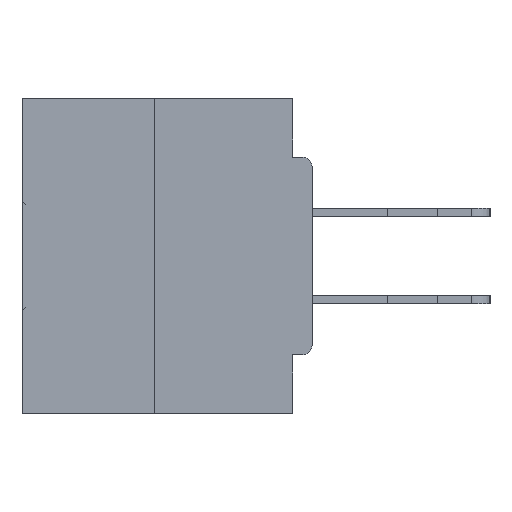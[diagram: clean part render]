
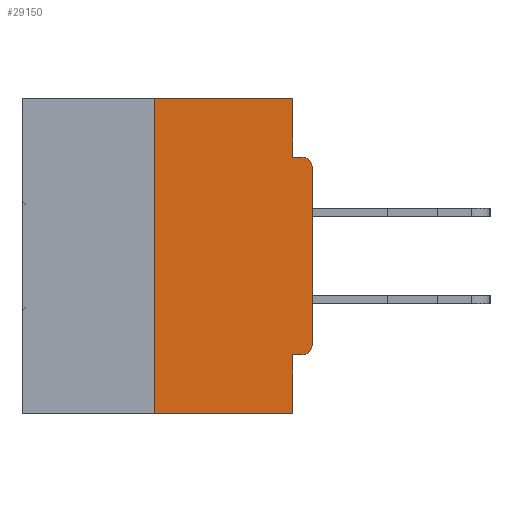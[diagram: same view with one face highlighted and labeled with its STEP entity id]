
A CAD part, left-side view. The second image highlights one B-rep face of the part: STEP entity #29150.
In plain terms, the highlighted planar face has unit normal (-1, 0, 0).
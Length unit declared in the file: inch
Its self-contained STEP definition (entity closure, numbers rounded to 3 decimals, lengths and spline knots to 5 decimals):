
#757 = DIRECTION ( 'NONE',  ( 0., -1., 0. ) ) ;
#1278 = CIRCLE ( 'NONE', #42327, 0.015 ) ;
#1602 = ORIENTED_EDGE ( 'NONE', *, *, #27210, .F. ) ;
#1636 = EDGE_CURVE ( 'NONE', #23093, #5491, #30600, .T. ) ;
#1952 = EDGE_CURVE ( 'NONE', #10516, #39162, #7034, .T. ) ;
#2072 = ORIENTED_EDGE ( 'NONE', *, *, #35229, .F. ) ;
#2387 = AXIS2_PLACEMENT_3D ( 'NONE', #27157, #37615, #17773 ) ;
#2455 = ORIENTED_EDGE ( 'NONE', *, *, #2737, .T. ) ;
#2729 = VECTOR ( 'NONE', #42596, 39.37008 ) ;
#2737 = EDGE_CURVE ( 'NONE', #21508, #10516, #1278, .T. ) ;
#2863 = VERTEX_POINT ( 'NONE', #5063 ) ;
#3002 = ORIENTED_EDGE ( 'NONE', *, *, #21280, .T. ) ;
#3651 = VERTEX_POINT ( 'NONE', #10582 ) ;
#4447 = ORIENTED_EDGE ( 'NONE', *, *, #31917, .F. ) ;
#5063 = CARTESIAN_POINT ( 'NONE',  ( 0., 0.031, 0. ) ) ;
#5491 = VERTEX_POINT ( 'NONE', #40994 ) ;
#6511 = VECTOR ( 'NONE', #39997, 39.37008 ) ;
#6859 = LINE ( 'NONE', #15985, #2729 ) ;
#7034 = LINE ( 'NONE', #16592, #27003 ) ;
#7607 = EDGE_CURVE ( 'NONE', #2863, #28866, #36518, .T. ) ;
#8617 = EDGE_LOOP ( 'NONE', ( #8826, #2072, #14465, #14925, #1602, #2455, #38104, #3002, #4447, #17056 ) ) ;
#8826 = ORIENTED_EDGE ( 'NONE', *, *, #15378, .F. ) ;
#10353 = CARTESIAN_POINT ( 'NONE',  ( 0., 0., -0.0935 ) ) ;
#10482 = AXIS2_PLACEMENT_3D ( 'NONE', #31400, #14598, #38144 ) ;
#10505 = CARTESIAN_POINT ( 'NONE',  ( 0., 0.015, -0.0935 ) ) ;
#10516 = VERTEX_POINT ( 'NONE', #36383 ) ;
#10582 = CARTESIAN_POINT ( 'NONE',  ( 0., 0.25, 0. ) ) ;
#12379 = VECTOR ( 'NONE', #36850, 39.37008 ) ;
#13379 = CARTESIAN_POINT ( 'NONE',  ( 0., 0.015, -0.4065 ) ) ;
#13617 = LINE ( 'NONE', #10353, #39685 ) ;
#13798 = CARTESIAN_POINT ( 'NONE',  ( 0., 0.46, 0. ) ) ;
#14465 = ORIENTED_EDGE ( 'NONE', *, *, #1636, .T. ) ;
#14598 = DIRECTION ( 'NONE',  ( 1., 0., 0. ) ) ;
#14925 = ORIENTED_EDGE ( 'NONE', *, *, #26092, .F. ) ;
#15378 = EDGE_CURVE ( 'NONE', #3651, #2863, #29747, .T. ) ;
#15456 = FACE_OUTER_BOUND ( 'NONE', #8617, .T. ) ;
#15766 = VERTEX_POINT ( 'NONE', #10505 ) ;
#15985 = CARTESIAN_POINT ( 'NONE',  ( 0., 0., -0.4065 ) ) ;
#16009 = DIRECTION ( 'NONE',  ( 0., 0., -1. ) ) ;
#16583 = DIRECTION ( 'NONE',  ( -1., 0., 0. ) ) ;
#16592 = CARTESIAN_POINT ( 'NONE',  ( 0., 0., 0. ) ) ;
#16785 = CARTESIAN_POINT ( 'NONE',  ( 0., 0.031, -0.5 ) ) ;
#17056 = ORIENTED_EDGE ( 'NONE', *, *, #7607, .F. ) ;
#17773 = DIRECTION ( 'NONE',  ( 0., 0., -1. ) ) ;
#20346 = DIRECTION ( 'NONE',  ( 0., -1., 0. ) ) ;
#20566 = LINE ( 'NONE', #33906, #23176 ) ;
#21280 = EDGE_CURVE ( 'NONE', #39162, #15766, #28014, .T. ) ;
#21508 = VERTEX_POINT ( 'NONE', #13379 ) ;
#22176 = CARTESIAN_POINT ( 'NONE',  ( 0., 0.031, -0.4065 ) ) ;
#23093 = VERTEX_POINT ( 'NONE', #39073 ) ;
#23176 = VECTOR ( 'NONE', #40825, 39.37008 ) ;
#23393 = CARTESIAN_POINT ( 'NONE',  ( 0., 0.031, 0. ) ) ;
#25492 = PLANE ( 'NONE',  #10482 ) ;
#25754 = CARTESIAN_POINT ( 'NONE',  ( 0., 0., -0.1085 ) ) ;
#25979 = DIRECTION ( 'NONE',  ( 0., 0., -1. ) ) ;
#26092 = EDGE_CURVE ( 'NONE', #33043, #5491, #33377, .T. ) ;
#27003 = VECTOR ( 'NONE', #30340, 39.37008 ) ;
#27157 = CARTESIAN_POINT ( 'NONE',  ( 0., 0.015, -0.1085 ) ) ;
#27210 = EDGE_CURVE ( 'NONE', #21508, #33043, #6859, .T. ) ;
#27688 = VECTOR ( 'NONE', #757, 39.37008 ) ;
#28014 = CIRCLE ( 'NONE', #2387, 0.015 ) ;
#28866 = VERTEX_POINT ( 'NONE', #39502 ) ;
#29150 = ADVANCED_FACE ( 'NONE', ( #15456 ), #25492, .F. ) ;
#29747 = LINE ( 'NONE', #13798, #6511 ) ;
#30340 = DIRECTION ( 'NONE',  ( 0., 0., 1. ) ) ;
#30600 = LINE ( 'NONE', #39768, #27688 ) ;
#31400 = CARTESIAN_POINT ( 'NONE',  ( 0., 0.46, 0. ) ) ;
#31917 = EDGE_CURVE ( 'NONE', #28866, #15766, #13617, .T. ) ;
#33043 = VERTEX_POINT ( 'NONE', #22176 ) ;
#33377 = LINE ( 'NONE', #16785, #12379 ) ;
#33906 = CARTESIAN_POINT ( 'NONE',  ( 0., 0.25, 0. ) ) ;
#35101 = VECTOR ( 'NONE', #16009, 39.37008 ) ;
#35229 = EDGE_CURVE ( 'NONE', #23093, #3651, #20566, .T. ) ;
#36383 = CARTESIAN_POINT ( 'NONE',  ( 0., 0., -0.3915 ) ) ;
#36518 = LINE ( 'NONE', #23393, #35101 ) ;
#36650 = CARTESIAN_POINT ( 'NONE',  ( 0., 0.015, -0.3915 ) ) ;
#36850 = DIRECTION ( 'NONE',  ( 0., 0., -1. ) ) ;
#37615 = DIRECTION ( 'NONE',  ( -1., 0., 0. ) ) ;
#38104 = ORIENTED_EDGE ( 'NONE', *, *, #1952, .T. ) ;
#38144 = DIRECTION ( 'NONE',  ( 0., 0., -1. ) ) ;
#39073 = CARTESIAN_POINT ( 'NONE',  ( 0., 0.25, -0.5 ) ) ;
#39162 = VERTEX_POINT ( 'NONE', #25754 ) ;
#39502 = CARTESIAN_POINT ( 'NONE',  ( 0., 0.031, -0.0935 ) ) ;
#39685 = VECTOR ( 'NONE', #20346, 39.37008 ) ;
#39768 = CARTESIAN_POINT ( 'NONE',  ( 0., 0.46, -0.5 ) ) ;
#39997 = DIRECTION ( 'NONE',  ( 0., -1., 0. ) ) ;
#40825 = DIRECTION ( 'NONE',  ( 0., 0., 1. ) ) ;
#40994 = CARTESIAN_POINT ( 'NONE',  ( 0., 0.031, -0.5 ) ) ;
#42327 = AXIS2_PLACEMENT_3D ( 'NONE', #36650, #16583, #25979 ) ;
#42596 = DIRECTION ( 'NONE',  ( 0., 1., 0. ) ) ;
